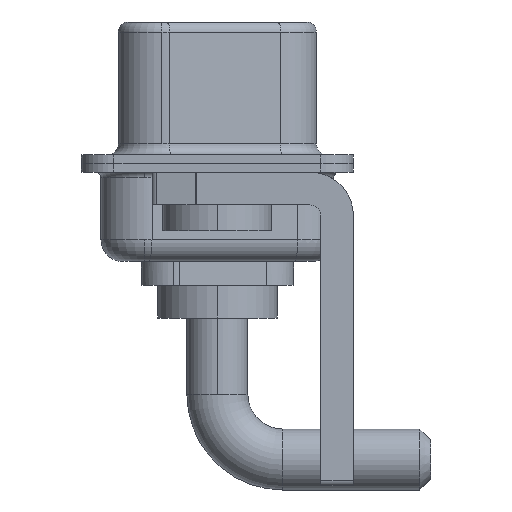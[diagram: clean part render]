
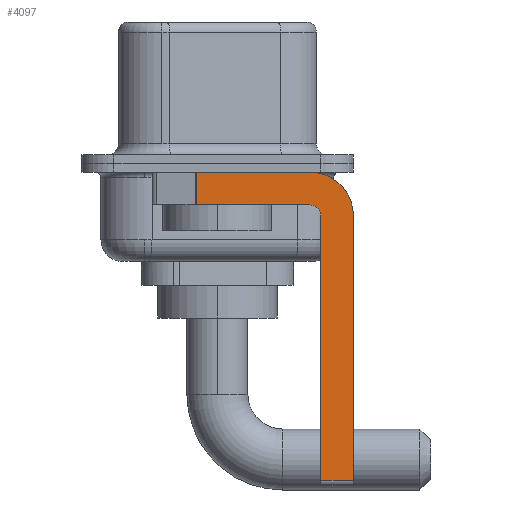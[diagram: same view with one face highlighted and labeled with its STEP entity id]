
A CAD part, left-side view. The second image highlights one B-rep face of the part: STEP entity #4097.
In plain terms, the highlighted planar face has unit normal (-1, 0, 0).
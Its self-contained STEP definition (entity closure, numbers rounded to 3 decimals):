
#113 = VERTEX_POINT ( 'NONE', #2164 ) ;
#368 = VERTEX_POINT ( 'NONE', #3785 ) ;
#431 = EDGE_CURVE ( 'NONE', #7065, #113, #9769, .T. ) ;
#519 = VECTOR ( 'NONE', #8956, 1000. ) ;
#713 = CARTESIAN_POINT ( 'NONE',  ( -2.9, 0.978, -1.9 ) ) ;
#795 = DIRECTION ( 'NONE',  ( -1., 0., 0. ) ) ;
#816 = CARTESIAN_POINT ( 'NONE',  ( -2.9, -4.75, -2.4 ) ) ;
#845 = VECTOR ( 'NONE', #12178, 1000. ) ;
#911 = VECTOR ( 'NONE', #4354, 1000. ) ;
#1023 = DIRECTION ( 'NONE',  ( 1., 0., 0. ) ) ;
#1117 = AXIS2_PLACEMENT_3D ( 'NONE', #11438, #795, #12965 ) ;
#1276 = CARTESIAN_POINT ( 'NONE',  ( -2.9, -6.25, -2.4 ) ) ;
#1476 = ORIENTED_EDGE ( 'NONE', *, *, #13953, .F. ) ;
#1504 = DIRECTION ( 'NONE',  ( 0., -1., 0. ) ) ;
#1603 = DIRECTION ( 'NONE',  ( 1., 0., 0. ) ) ;
#1902 = VECTOR ( 'NONE', #1504, 1000. ) ;
#2164 = CARTESIAN_POINT ( 'NONE',  ( -2.9, 0.978, -1.9 ) ) ;
#2551 = VERTEX_POINT ( 'NONE', #7487 ) ;
#2607 = CIRCLE ( 'NONE', #1117, 0.5 ) ;
#3131 = ORIENTED_EDGE ( 'NONE', *, *, #431, .F. ) ;
#3785 = CARTESIAN_POINT ( 'NONE',  ( -2.9, 0.978, -0.4 ) ) ;
#4097 = ADVANCED_FACE ( 'NONE', ( #8025 ), #4146, .F. ) ;
#4146 = PLANE ( 'NONE',  #13533 ) ;
#4354 = DIRECTION ( 'NONE',  ( 0., 0., -1. ) ) ;
#5031 = EDGE_CURVE ( 'NONE', #368, #8294, #12145, .T. ) ;
#5198 = ORIENTED_EDGE ( 'NONE', *, *, #5031, .F. ) ;
#5302 = ORIENTED_EDGE ( 'NONE', *, *, #5671, .T. ) ;
#5455 = CARTESIAN_POINT ( 'NONE',  ( -2.9, -4.75, -14.8 ) ) ;
#5671 = EDGE_CURVE ( 'NONE', #368, #113, #7707, .T. ) ;
#6320 = DIRECTION ( 'NONE',  ( 0., 0., -1. ) ) ;
#6652 = VERTEX_POINT ( 'NONE', #816 ) ;
#6959 = EDGE_CURVE ( 'NONE', #11206, #2551, #10904, .T. ) ;
#7065 = VERTEX_POINT ( 'NONE', #10979 ) ;
#7373 = CARTESIAN_POINT ( 'NONE',  ( -2.9, -6.25, -2.4 ) ) ;
#7487 = CARTESIAN_POINT ( 'NONE',  ( -2.9, -6.25, -14.55 ) ) ;
#7553 = AXIS2_PLACEMENT_3D ( 'NONE', #10920, #1603, #10085 ) ;
#7707 = LINE ( 'NONE', #713, #911 ) ;
#8025 = FACE_OUTER_BOUND ( 'NONE', #13832, .T. ) ;
#8049 = ORIENTED_EDGE ( 'NONE', *, *, #14894, .F. ) ;
#8294 = VERTEX_POINT ( 'NONE', #13325 ) ;
#8956 = DIRECTION ( 'NONE',  ( 0., 0., 1. ) ) ;
#9769 = LINE ( 'NONE', #11173, #845 ) ;
#9899 = EDGE_CURVE ( 'NONE', #14959, #6652, #10429, .T. ) ;
#10085 = DIRECTION ( 'NONE',  ( 0., 0., -1. ) ) ;
#10261 = LINE ( 'NONE', #13891, #13692 ) ;
#10429 = LINE ( 'NONE', #5455, #519 ) ;
#10904 = LINE ( 'NONE', #1276, #15326 ) ;
#10920 = CARTESIAN_POINT ( 'NONE',  ( -2.9, -4.25, -2.4 ) ) ;
#10979 = CARTESIAN_POINT ( 'NONE',  ( -2.9, -4.25, -1.9 ) ) ;
#11103 = ORIENTED_EDGE ( 'NONE', *, *, #11360, .T. ) ;
#11173 = CARTESIAN_POINT ( 'NONE',  ( -2.9, -4.25, -1.9 ) ) ;
#11206 = VERTEX_POINT ( 'NONE', #7373 ) ;
#11215 = CARTESIAN_POINT ( 'NONE',  ( -2.9, 3., -0.4 ) ) ;
#11360 = EDGE_CURVE ( 'NONE', #14959, #2551, #10261, .T. ) ;
#11438 = CARTESIAN_POINT ( 'NONE',  ( -2.9, -4.25, -2.4 ) ) ;
#11440 = ORIENTED_EDGE ( 'NONE', *, *, #6959, .F. ) ;
#12145 = LINE ( 'NONE', #11215, #1902 ) ;
#12178 = DIRECTION ( 'NONE',  ( 0., 1., 0. ) ) ;
#12677 = CARTESIAN_POINT ( 'NONE',  ( -2.9, -4.75, -14.55 ) ) ;
#12965 = DIRECTION ( 'NONE',  ( 0., 0., 1. ) ) ;
#13325 = CARTESIAN_POINT ( 'NONE',  ( -2.9, -4.25, -0.4 ) ) ;
#13533 = AXIS2_PLACEMENT_3D ( 'NONE', #15229, #1023, #14208 ) ;
#13692 = VECTOR ( 'NONE', #14984, 1000. ) ;
#13736 = CIRCLE ( 'NONE', #7553, 2. ) ;
#13832 = EDGE_LOOP ( 'NONE', ( #5198, #5302, #3131, #8049, #14597, #11103, #11440, #1476 ) ) ;
#13891 = CARTESIAN_POINT ( 'NONE',  ( -2.9, -4.25, -14.55 ) ) ;
#13953 = EDGE_CURVE ( 'NONE', #8294, #11206, #13736, .T. ) ;
#14208 = DIRECTION ( 'NONE',  ( 0., 0., -1. ) ) ;
#14597 = ORIENTED_EDGE ( 'NONE', *, *, #9899, .F. ) ;
#14894 = EDGE_CURVE ( 'NONE', #6652, #7065, #2607, .T. ) ;
#14959 = VERTEX_POINT ( 'NONE', #12677 ) ;
#14984 = DIRECTION ( 'NONE',  ( 0., -1., 0. ) ) ;
#15229 = CARTESIAN_POINT ( 'NONE',  ( -2.9, -4.25, -2.4 ) ) ;
#15326 = VECTOR ( 'NONE', #6320, 1000. ) ;
